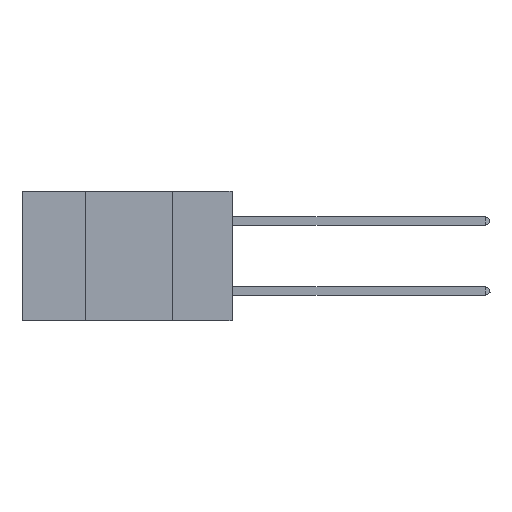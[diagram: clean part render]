
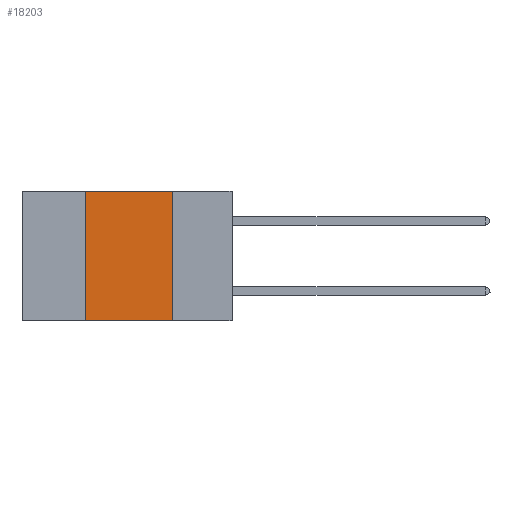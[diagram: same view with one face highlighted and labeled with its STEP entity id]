
A CAD part, left-side view. The second image highlights one B-rep face of the part: STEP entity #18203.
In plain terms, the highlighted planar face has unit normal (-1, 0, 0).
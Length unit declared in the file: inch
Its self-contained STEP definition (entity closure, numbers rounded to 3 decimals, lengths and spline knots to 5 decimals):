
#580 = CARTESIAN_POINT ( 'NONE',  ( 0., 0.42, 0. ) ) ;
#754 = FACE_OUTER_BOUND ( 'NONE', #4219, .T. ) ;
#1861 = DIRECTION ( 'NONE',  ( 0., -1., 0. ) ) ;
#1863 = CARTESIAN_POINT ( 'NONE',  ( 0., 0.17, -0.37 ) ) ;
#1897 = LINE ( 'NONE', #16193, #26912 ) ;
#4219 = EDGE_LOOP ( 'NONE', ( #9356, #9911, #13709, #20444 ) ) ;
#5490 = CARTESIAN_POINT ( 'NONE',  ( 0., 0.17, 0. ) ) ;
#5844 = EDGE_CURVE ( 'NONE', #5969, #12292, #1897, .T. ) ;
#5969 = VERTEX_POINT ( 'NONE', #580 ) ;
#8911 = VECTOR ( 'NONE', #1861, 39.37008 ) ;
#9356 = ORIENTED_EDGE ( 'NONE', *, *, #13830, .F. ) ;
#9911 = ORIENTED_EDGE ( 'NONE', *, *, #5844, .F. ) ;
#10387 = DIRECTION ( 'NONE',  ( 0., 0., 1. ) ) ;
#11189 = LINE ( 'NONE', #18869, #15751 ) ;
#11892 = VECTOR ( 'NONE', #10387, 39.37008 ) ;
#12198 = CARTESIAN_POINT ( 'NONE',  ( 0., 0.42, -0.37 ) ) ;
#12292 = VERTEX_POINT ( 'NONE', #5490 ) ;
#13709 = ORIENTED_EDGE ( 'NONE', *, *, #23773, .F. ) ;
#13790 = EDGE_CURVE ( 'NONE', #26043, #22516, #25681, .T. ) ;
#13830 = EDGE_CURVE ( 'NONE', #12292, #22516, #11189, .T. ) ;
#14342 = DIRECTION ( 'NONE',  ( 1., 0., 0. ) ) ;
#15751 = VECTOR ( 'NONE', #18687, 39.37008 ) ;
#16089 = CARTESIAN_POINT ( 'NONE',  ( 0., 0.6, 0. ) ) ;
#16193 = CARTESIAN_POINT ( 'NONE',  ( 0., 0.6, 0. ) ) ;
#16365 = PLANE ( 'NONE',  #27026 ) ;
#18203 = ADVANCED_FACE ( 'NONE', ( #754 ), #16365, .F. ) ;
#18542 = DIRECTION ( 'NONE',  ( 0., -1., 0. ) ) ;
#18687 = DIRECTION ( 'NONE',  ( 0., 0., -1. ) ) ;
#18869 = CARTESIAN_POINT ( 'NONE',  ( 0., 0.17, 0. ) ) ;
#18965 = CARTESIAN_POINT ( 'NONE',  ( 0., 0.42, 0. ) ) ;
#20444 = ORIENTED_EDGE ( 'NONE', *, *, #13790, .T. ) ;
#22516 = VERTEX_POINT ( 'NONE', #1863 ) ;
#22574 = DIRECTION ( 'NONE',  ( 0., 0., -1. ) ) ;
#23773 = EDGE_CURVE ( 'NONE', #26043, #5969, #24685, .T. ) ;
#24685 = LINE ( 'NONE', #18965, #11892 ) ;
#25661 = CARTESIAN_POINT ( 'NONE',  ( 0., 0.6, -0.37 ) ) ;
#25681 = LINE ( 'NONE', #25661, #8911 ) ;
#26043 = VERTEX_POINT ( 'NONE', #12198 ) ;
#26912 = VECTOR ( 'NONE', #18542, 39.37008 ) ;
#27026 = AXIS2_PLACEMENT_3D ( 'NONE', #16089, #14342, #22574 ) ;
